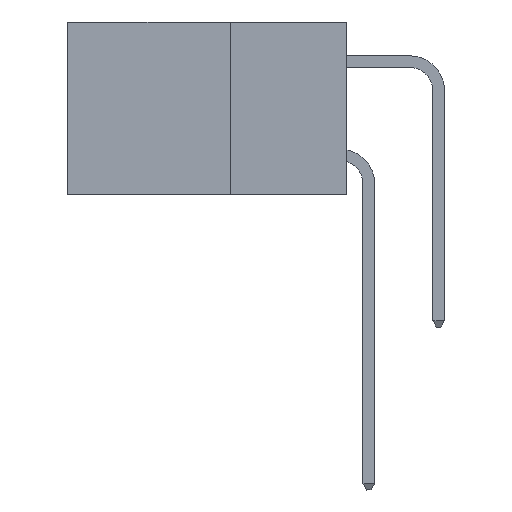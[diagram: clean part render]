
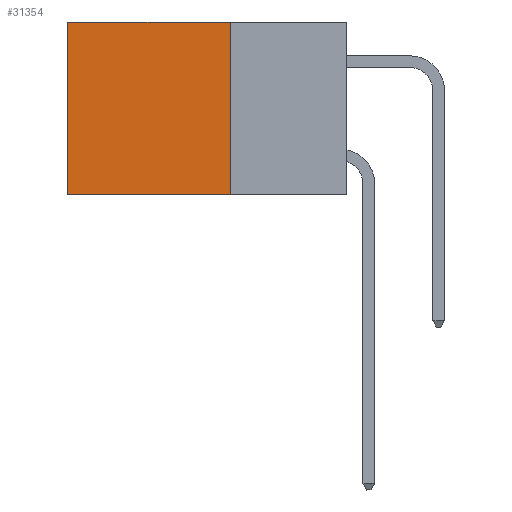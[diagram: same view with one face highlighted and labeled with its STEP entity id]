
A CAD part, left-side view. The second image highlights one B-rep face of the part: STEP entity #31354.
In plain terms, the highlighted planar face has unit normal (-1, 0, 0).
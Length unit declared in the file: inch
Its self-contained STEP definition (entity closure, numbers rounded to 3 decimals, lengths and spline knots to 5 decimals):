
#97 = ORIENTED_EDGE ( 'NONE', *, *, #31368, .T. ) ;
#2104 = CARTESIAN_POINT ( 'NONE',  ( 0.2875, 0.25, 0. ) ) ;
#3780 = CARTESIAN_POINT ( 'NONE',  ( 0.2875, 0.25, -0.37 ) ) ;
#6857 = VERTEX_POINT ( 'NONE', #25643 ) ;
#7194 = CARTESIAN_POINT ( 'NONE',  ( 0.2875, 0.25, 0. ) ) ;
#9319 = VERTEX_POINT ( 'NONE', #13355 ) ;
#9533 = ORIENTED_EDGE ( 'NONE', *, *, #23489, .T. ) ;
#9906 = LINE ( 'NONE', #2104, #40699 ) ;
#10163 = CARTESIAN_POINT ( 'NONE',  ( 0.2875, 0.6, 0. ) ) ;
#11355 = EDGE_LOOP ( 'NONE', ( #97, #24767, #21290, #9533 ) ) ;
#13098 = DIRECTION ( 'NONE',  ( 0., 1., 0. ) ) ;
#13104 = DIRECTION ( 'NONE',  ( 0., 1., 0. ) ) ;
#13355 = CARTESIAN_POINT ( 'NONE',  ( 0.2875, 0.25, -0.37 ) ) ;
#13849 = DIRECTION ( 'NONE',  ( 0., 0., -1. ) ) ;
#16811 = EDGE_CURVE ( 'NONE', #19299, #9319, #9906, .T. ) ;
#18121 = AXIS2_PLACEMENT_3D ( 'NONE', #7194, #29820, #39497 ) ;
#19299 = VERTEX_POINT ( 'NONE', #32136 ) ;
#21290 = ORIENTED_EDGE ( 'NONE', *, *, #16811, .F. ) ;
#22064 = VECTOR ( 'NONE', #13104, 39.37008 ) ;
#23011 = LINE ( 'NONE', #10163, #25571 ) ;
#23489 = EDGE_CURVE ( 'NONE', #19299, #6857, #37043, .T. ) ;
#24767 = ORIENTED_EDGE ( 'NONE', *, *, #30175, .F. ) ;
#25091 = CARTESIAN_POINT ( 'NONE',  ( 0.2875, 0.25, 0. ) ) ;
#25571 = VECTOR ( 'NONE', #13849, 39.37008 ) ;
#25643 = CARTESIAN_POINT ( 'NONE',  ( 0.2875, 0.6, 0. ) ) ;
#29304 = VERTEX_POINT ( 'NONE', #34644 ) ;
#29414 = PLANE ( 'NONE',  #18121 ) ;
#29820 = DIRECTION ( 'NONE',  ( 1., 0., 0. ) ) ;
#30175 = EDGE_CURVE ( 'NONE', #9319, #29304, #39696, .T. ) ;
#31354 = ADVANCED_FACE ( 'NONE', ( #39142 ), #29414, .F. ) ;
#31368 = EDGE_CURVE ( 'NONE', #6857, #29304, #23011, .T. ) ;
#32136 = CARTESIAN_POINT ( 'NONE',  ( 0.2875, 0.25, 0. ) ) ;
#32541 = VECTOR ( 'NONE', #13098, 39.37008 ) ;
#34002 = DIRECTION ( 'NONE',  ( 0., 0., -1. ) ) ;
#34644 = CARTESIAN_POINT ( 'NONE',  ( 0.2875, 0.6, -0.37 ) ) ;
#37043 = LINE ( 'NONE', #25091, #32541 ) ;
#39142 = FACE_OUTER_BOUND ( 'NONE', #11355, .T. ) ;
#39497 = DIRECTION ( 'NONE',  ( 0., 0., -1. ) ) ;
#39696 = LINE ( 'NONE', #3780, #22064 ) ;
#40699 = VECTOR ( 'NONE', #34002, 39.37008 ) ;
